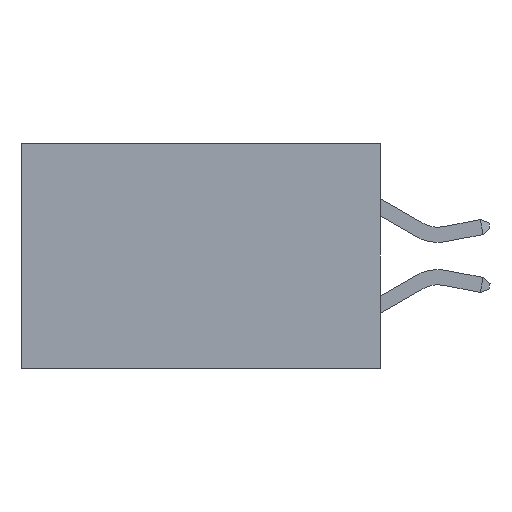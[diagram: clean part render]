
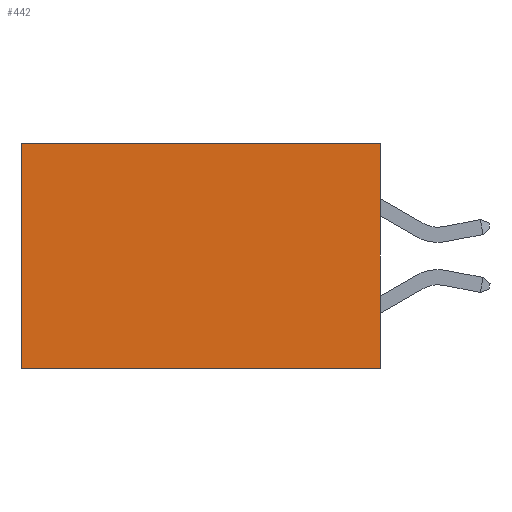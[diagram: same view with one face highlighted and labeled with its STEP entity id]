
A CAD part, left-side view. The second image highlights one B-rep face of the part: STEP entity #442.
In plain terms, the highlighted planar face has unit normal (-1, 0, 0).
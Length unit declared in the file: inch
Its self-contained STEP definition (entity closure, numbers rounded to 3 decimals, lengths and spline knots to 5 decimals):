
#102 = ORIENTED_EDGE ( 'NONE', *, *, #2974, .F. ) ;
#213 = DIRECTION ( 'NONE',  ( 0., 1., 0. ) ) ;
#442 = ADVANCED_FACE ( 'NONE', ( #12071 ), #14141, .F. ) ;
#808 = LINE ( 'NONE', #1453, #6326 ) ;
#841 = CARTESIAN_POINT ( 'NONE',  ( 0.277, 0., -0.37 ) ) ;
#890 = EDGE_CURVE ( 'NONE', #12589, #5145, #1458, .T. ) ;
#1453 = CARTESIAN_POINT ( 'NONE',  ( 0.277, 0., -0.37 ) ) ;
#1458 = LINE ( 'NONE', #11908, #13370 ) ;
#1540 = DIRECTION ( 'NONE',  ( 0., 1., 0. ) ) ;
#2432 = EDGE_CURVE ( 'NONE', #13244, #12589, #3959, .T. ) ;
#2974 = EDGE_CURVE ( 'NONE', #13244, #6077, #12168, .T. ) ;
#3228 = VECTOR ( 'NONE', #213, 39.37008 ) ;
#3959 = LINE ( 'NONE', #6295, #3228 ) ;
#4474 = CARTESIAN_POINT ( 'NONE',  ( 0.277, 0.59, 0. ) ) ;
#4599 = CARTESIAN_POINT ( 'NONE',  ( 0.277, 0., -0.37 ) ) ;
#5145 = VERTEX_POINT ( 'NONE', #6635 ) ;
#6077 = VERTEX_POINT ( 'NONE', #4599 ) ;
#6295 = CARTESIAN_POINT ( 'NONE',  ( 0.277, 0., 0. ) ) ;
#6326 = VECTOR ( 'NONE', #1540, 39.37008 ) ;
#6635 = CARTESIAN_POINT ( 'NONE',  ( 0.277, 0.59, -0.37 ) ) ;
#6733 = ORIENTED_EDGE ( 'NONE', *, *, #2432, .T. ) ;
#7596 = EDGE_CURVE ( 'NONE', #6077, #5145, #808, .T. ) ;
#8272 = CARTESIAN_POINT ( 'NONE',  ( 0.277, 0., -0.37 ) ) ;
#8774 = DIRECTION ( 'NONE',  ( 0., 0., -1. ) ) ;
#9245 = VECTOR ( 'NONE', #13379, 39.37008 ) ;
#9417 = AXIS2_PLACEMENT_3D ( 'NONE', #841, #14126, #8774 ) ;
#10859 = ORIENTED_EDGE ( 'NONE', *, *, #890, .T. ) ;
#11086 = CARTESIAN_POINT ( 'NONE',  ( 0.277, 0., 0. ) ) ;
#11736 = DIRECTION ( 'NONE',  ( 0., 0., -1. ) ) ;
#11908 = CARTESIAN_POINT ( 'NONE',  ( 0.277, 0.59, -0.37 ) ) ;
#12071 = FACE_OUTER_BOUND ( 'NONE', #12383, .T. ) ;
#12168 = LINE ( 'NONE', #8272, #9245 ) ;
#12383 = EDGE_LOOP ( 'NONE', ( #10859, #13686, #102, #6733 ) ) ;
#12589 = VERTEX_POINT ( 'NONE', #4474 ) ;
#13244 = VERTEX_POINT ( 'NONE', #11086 ) ;
#13370 = VECTOR ( 'NONE', #11736, 39.37008 ) ;
#13379 = DIRECTION ( 'NONE',  ( 0., 0., -1. ) ) ;
#13686 = ORIENTED_EDGE ( 'NONE', *, *, #7596, .F. ) ;
#14126 = DIRECTION ( 'NONE',  ( 1., 0., 0. ) ) ;
#14141 = PLANE ( 'NONE',  #9417 ) ;
